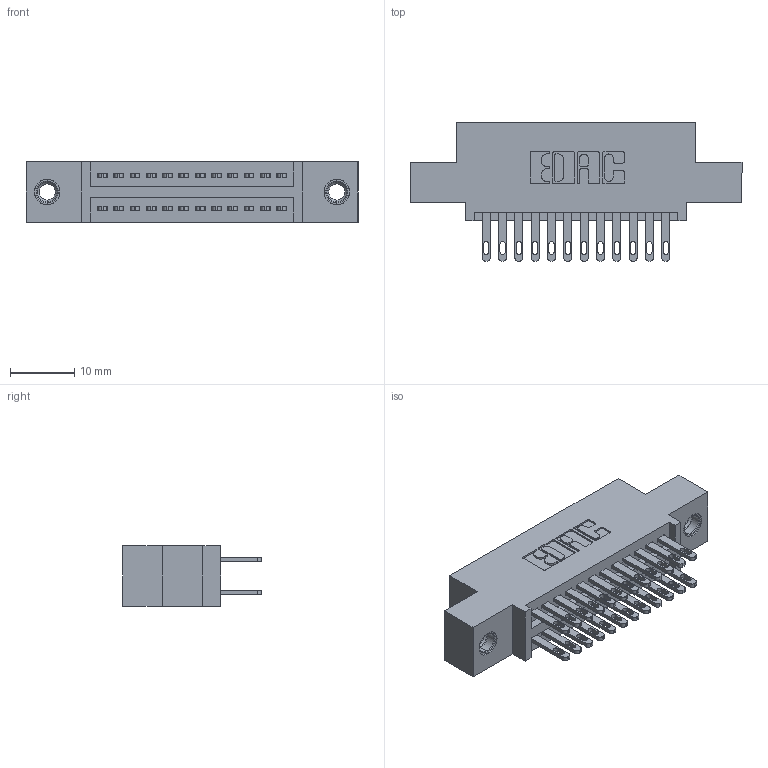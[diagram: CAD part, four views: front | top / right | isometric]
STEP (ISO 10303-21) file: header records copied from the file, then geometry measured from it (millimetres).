
FILE_DESCRIPTION (( 'STEP AP203' ), '1' );
FILE_NAME ('895-024-500-507.STEP', '2020-09-25T13:02:23', ( '' ), ( '' ), 'SwSTEP 2.0', 'SolidWorks 2020', '' );
FILE_SCHEMA (( 'CONFIG_CONTROL_DESIGN' ));
Length unit declared in the file: inch
Products named in the file (4): 845 Part_0.110 Offset - 0.156 Dia-TI; 345-250-001_345-250-005-103; 345-292-001_345-293-100; 895-024-500-507
Assembly tree (27 placements, depth 2):
  895-024-500-507
    845 Part_0.110 Offset - 0.156 Dia-TI
    345-292-001_345-293-100  x24
    345-250-001_345-250-005-103  x2
Bounding box: 51.69 x 21.51 x 9.4 mm (x, y, z)
Volume: 4729.1 mm3; surface area: 6774.9 mm2
Topology: 27 solids, 27 shells, 1294 faces, 3873 edges, 2574 vertices
Faces by surface type: plane 764, cylinder 514, cone 12, torus 4
Entity records: 14702 total; most frequent: CARTESIAN_POINT 2475, ORIENTED_EDGE 2402, DIRECTION 2247, EDGE_CURVE 1201, LINE 997, VECTOR 997, VERTEX_POINT 796, AXIS2_PLACEMENT_3D 625
